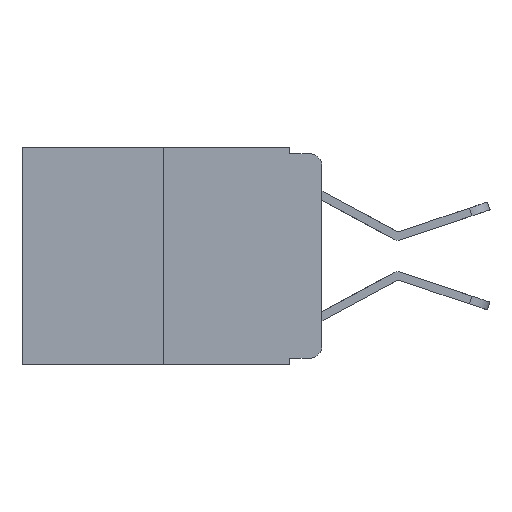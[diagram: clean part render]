
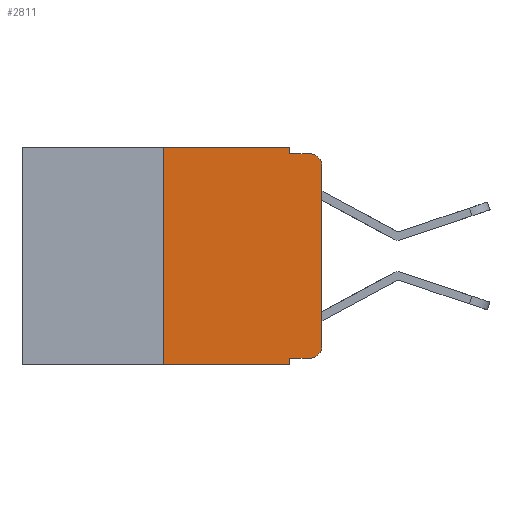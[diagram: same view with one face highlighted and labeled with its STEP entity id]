
A CAD part, left-side view. The second image highlights one B-rep face of the part: STEP entity #2811.
In plain terms, the highlighted planar face has unit normal (-1, 0, 0).
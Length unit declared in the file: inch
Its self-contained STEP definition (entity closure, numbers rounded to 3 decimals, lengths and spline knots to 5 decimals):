
#110 = CARTESIAN_POINT ( 'NONE',  ( 0., 0., 0. ) ) ;
#260 = EDGE_CURVE ( 'NONE', #8026, #6965, #889, .T. ) ;
#522 = CARTESIAN_POINT ( 'NONE',  ( 0., 0.051, -0.343 ) ) ;
#730 = AXIS2_PLACEMENT_3D ( 'NONE', #7097, #7240, #7231 ) ;
#812 = DIRECTION ( 'NONE',  ( 0., -1., 0. ) ) ;
#889 = LINE ( 'NONE', #2036, #8938 ) ;
#997 = LINE ( 'NONE', #8924, #3353 ) ;
#1208 = DIRECTION ( 'NONE',  ( 0., -1., 0. ) ) ;
#1250 = DIRECTION ( 'NONE',  ( 0., 0., 1. ) ) ;
#1404 = DIRECTION ( 'NONE',  ( 0., 0., -1. ) ) ;
#1423 = EDGE_CURVE ( 'NONE', #6965, #4835, #9143, .T. ) ;
#1435 = CARTESIAN_POINT ( 'NONE',  ( 0., 0.02, -0.313 ) ) ;
#1470 = DIRECTION ( 'NONE',  ( -1., 0., 0. ) ) ;
#1631 = ORIENTED_EDGE ( 'NONE', *, *, #2630, .T. ) ;
#1696 = VECTOR ( 'NONE', #2433, 39.37008 ) ;
#1826 = DIRECTION ( 'NONE',  ( 0., 0., -1. ) ) ;
#1961 = VECTOR ( 'NONE', #8380, 39.37008 ) ;
#2036 = CARTESIAN_POINT ( 'NONE',  ( 0., 0.051, 0. ) ) ;
#2047 = EDGE_CURVE ( 'NONE', #4471, #4835, #5129, .T. ) ;
#2225 = VERTEX_POINT ( 'NONE', #8515 ) ;
#2295 = ORIENTED_EDGE ( 'NONE', *, *, #260, .F. ) ;
#2433 = DIRECTION ( 'NONE',  ( 0., -1., 0. ) ) ;
#2508 = ORIENTED_EDGE ( 'NONE', *, *, #7641, .T. ) ;
#2540 = CARTESIAN_POINT ( 'NONE',  ( 0., 0.473, -0.343 ) ) ;
#2630 = EDGE_CURVE ( 'NONE', #9969, #4471, #6193, .T. ) ;
#2795 = LINE ( 'NONE', #3187, #5003 ) ;
#2811 = ADVANCED_FACE ( 'NONE', ( #6785 ), #6538, .F. ) ;
#3023 = ORIENTED_EDGE ( 'NONE', *, *, #8890, .F. ) ;
#3055 = CARTESIAN_POINT ( 'NONE',  ( 0., 0.25, 0. ) ) ;
#3138 = CARTESIAN_POINT ( 'NONE',  ( 0., 0.051, -0.333 ) ) ;
#3187 = CARTESIAN_POINT ( 'NONE',  ( 0., 0.051, 0. ) ) ;
#3353 = VECTOR ( 'NONE', #8490, 39.37008 ) ;
#3592 = CARTESIAN_POINT ( 'NONE',  ( 0., 0., -0.313 ) ) ;
#3748 = VERTEX_POINT ( 'NONE', #8090 ) ;
#3829 = ORIENTED_EDGE ( 'NONE', *, *, #2047, .T. ) ;
#4003 = EDGE_CURVE ( 'NONE', #3748, #9969, #7485, .T. ) ;
#4144 = VECTOR ( 'NONE', #1250, 39.37008 ) ;
#4237 = DIRECTION ( 'NONE',  ( 0., 0., -1. ) ) ;
#4317 = VERTEX_POINT ( 'NONE', #3138 ) ;
#4471 = VERTEX_POINT ( 'NONE', #8316 ) ;
#4486 = CARTESIAN_POINT ( 'NONE',  ( 0., 0.02, -0.01 ) ) ;
#4552 = ORIENTED_EDGE ( 'NONE', *, *, #8535, .F. ) ;
#4835 = VERTEX_POINT ( 'NONE', #4486 ) ;
#5003 = VECTOR ( 'NONE', #8487, 39.37008 ) ;
#5129 = CIRCLE ( 'NONE', #6388, 0.02 ) ;
#5192 = VERTEX_POINT ( 'NONE', #522 ) ;
#5383 = VECTOR ( 'NONE', #1208, 39.37008 ) ;
#6193 = LINE ( 'NONE', #110, #4144 ) ;
#6376 = ORIENTED_EDGE ( 'NONE', *, *, #6610, .T. ) ;
#6388 = AXIS2_PLACEMENT_3D ( 'NONE', #7838, #7624, #4237 ) ;
#6538 = PLANE ( 'NONE',  #730 ) ;
#6579 = VECTOR ( 'NONE', #812, 39.37008 ) ;
#6610 = EDGE_CURVE ( 'NONE', #4317, #3748, #997, .T. ) ;
#6613 = CARTESIAN_POINT ( 'NONE',  ( 0., 0.473, 0. ) ) ;
#6785 = FACE_OUTER_BOUND ( 'NONE', #9069, .T. ) ;
#6899 = LINE ( 'NONE', #6613, #6579 ) ;
#6915 = CARTESIAN_POINT ( 'NONE',  ( 0., 0.051, -0.01 ) ) ;
#6965 = VERTEX_POINT ( 'NONE', #7022 ) ;
#7022 = CARTESIAN_POINT ( 'NONE',  ( 0., 0.051, -0.01 ) ) ;
#7097 = CARTESIAN_POINT ( 'NONE',  ( 0., 0.473, 0. ) ) ;
#7231 = DIRECTION ( 'NONE',  ( 0., 0., -1. ) ) ;
#7240 = DIRECTION ( 'NONE',  ( 1., 0., 0. ) ) ;
#7266 = ORIENTED_EDGE ( 'NONE', *, *, #4003, .T. ) ;
#7312 = CARTESIAN_POINT ( 'NONE',  ( 0., 0.25, 0. ) ) ;
#7361 = VERTEX_POINT ( 'NONE', #7312 ) ;
#7485 = CIRCLE ( 'NONE', #7672, 0.02 ) ;
#7586 = ORIENTED_EDGE ( 'NONE', *, *, #1423, .F. ) ;
#7624 = DIRECTION ( 'NONE',  ( -1., 0., 0. ) ) ;
#7641 = EDGE_CURVE ( 'NONE', #2225, #5192, #9356, .T. ) ;
#7651 = ORIENTED_EDGE ( 'NONE', *, *, #9347, .F. ) ;
#7672 = AXIS2_PLACEMENT_3D ( 'NONE', #1435, #1470, #1404 ) ;
#7838 = CARTESIAN_POINT ( 'NONE',  ( 0., 0.02, -0.03 ) ) ;
#7954 = LINE ( 'NONE', #3055, #1961 ) ;
#8026 = VERTEX_POINT ( 'NONE', #9625 ) ;
#8090 = CARTESIAN_POINT ( 'NONE',  ( 0., 0.02, -0.333 ) ) ;
#8316 = CARTESIAN_POINT ( 'NONE',  ( 0., 0., -0.03 ) ) ;
#8380 = DIRECTION ( 'NONE',  ( 0., 0., 1. ) ) ;
#8487 = DIRECTION ( 'NONE',  ( 0., 0., -1. ) ) ;
#8490 = DIRECTION ( 'NONE',  ( 0., -1., 0. ) ) ;
#8515 = CARTESIAN_POINT ( 'NONE',  ( 0., 0.25, -0.343 ) ) ;
#8535 = EDGE_CURVE ( 'NONE', #7361, #8026, #6899, .T. ) ;
#8890 = EDGE_CURVE ( 'NONE', #4317, #5192, #2795, .T. ) ;
#8924 = CARTESIAN_POINT ( 'NONE',  ( 0., 0.051, -0.333 ) ) ;
#8938 = VECTOR ( 'NONE', #1826, 39.37008 ) ;
#9069 = EDGE_LOOP ( 'NONE', ( #1631, #3829, #7586, #2295, #4552, #7651, #2508, #3023, #6376, #7266 ) ) ;
#9143 = LINE ( 'NONE', #6915, #5383 ) ;
#9347 = EDGE_CURVE ( 'NONE', #2225, #7361, #7954, .T. ) ;
#9356 = LINE ( 'NONE', #2540, #1696 ) ;
#9625 = CARTESIAN_POINT ( 'NONE',  ( 0., 0.051, 0. ) ) ;
#9969 = VERTEX_POINT ( 'NONE', #3592 ) ;
